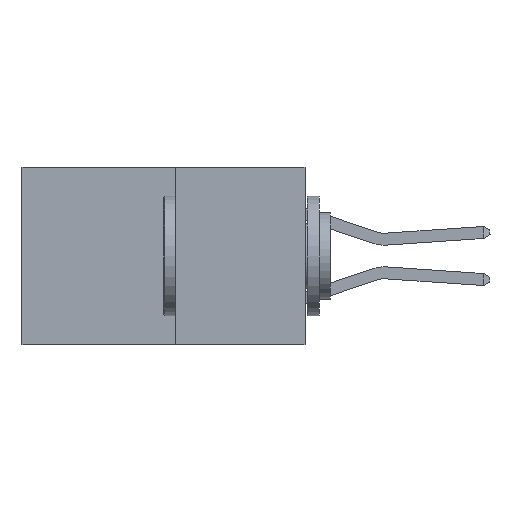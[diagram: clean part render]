
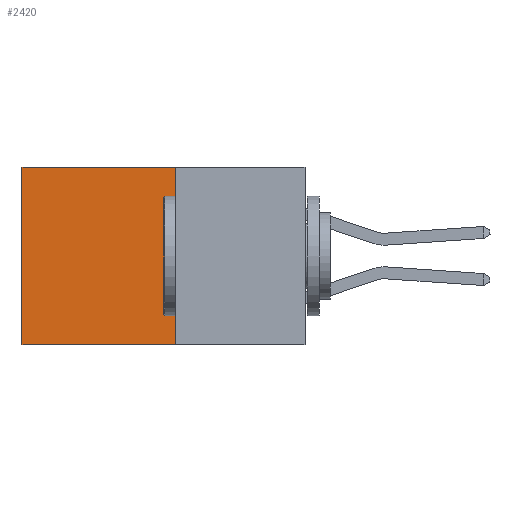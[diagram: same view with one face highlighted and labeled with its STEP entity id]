
A CAD part, left-side view. The second image highlights one B-rep face of the part: STEP entity #2420.
In plain terms, the highlighted planar face has unit normal (-1, 0, 0).
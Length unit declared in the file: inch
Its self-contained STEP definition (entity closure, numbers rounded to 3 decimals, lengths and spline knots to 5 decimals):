
#231 = CARTESIAN_POINT ( 'NONE',  ( 0.277, 0.27, 0. ) ) ;
#305 = LINE ( 'NONE', #4932, #8476 ) ;
#580 = DIRECTION ( 'NONE',  ( 0., 1., 0. ) ) ;
#593 = ORIENTED_EDGE ( 'NONE', *, *, #9528, .F. ) ;
#755 = DIRECTION ( 'NONE',  ( 0., 1., 0. ) ) ;
#769 = CARTESIAN_POINT ( 'NONE',  ( 0.277, 0.27, -0.37 ) ) ;
#1310 = CARTESIAN_POINT ( 'NONE',  ( 0.277, 0.27, -0.37 ) ) ;
#2315 = FACE_OUTER_BOUND ( 'NONE', #2800, .T. ) ;
#2420 = ADVANCED_FACE ( 'NONE', ( #2315 ), #5963, .F. ) ;
#2690 = LINE ( 'NONE', #1310, #4550 ) ;
#2800 = EDGE_LOOP ( 'NONE', ( #2806, #593, #2823, #6889 ) ) ;
#2801 = EDGE_CURVE ( 'NONE', #5486, #8533, #305, .T. ) ;
#2806 = ORIENTED_EDGE ( 'NONE', *, *, #2801, .T. ) ;
#2823 = ORIENTED_EDGE ( 'NONE', *, *, #6991, .F. ) ;
#3002 = VECTOR ( 'NONE', #580, 39.37008 ) ;
#3126 = DIRECTION ( 'NONE',  ( 0., 0., -1. ) ) ;
#3363 = DIRECTION ( 'NONE',  ( 0., 0., -1. ) ) ;
#3521 = CARTESIAN_POINT ( 'NONE',  ( 0.277, 0.59, 0. ) ) ;
#3761 = CARTESIAN_POINT ( 'NONE',  ( 0.277, 0.59, -0.37 ) ) ;
#3811 = EDGE_CURVE ( 'NONE', #9253, #5486, #9293, .T. ) ;
#4550 = VECTOR ( 'NONE', #3126, 39.37008 ) ;
#4932 = CARTESIAN_POINT ( 'NONE',  ( 0.277, 0.59, -0.37 ) ) ;
#5310 = DIRECTION ( 'NONE',  ( 0., 0., -1. ) ) ;
#5486 = VERTEX_POINT ( 'NONE', #3521 ) ;
#5963 = PLANE ( 'NONE',  #9778 ) ;
#6267 = VERTEX_POINT ( 'NONE', #8669 ) ;
#6889 = ORIENTED_EDGE ( 'NONE', *, *, #3811, .T. ) ;
#6991 = EDGE_CURVE ( 'NONE', #9253, #6267, #2690, .T. ) ;
#7345 = VECTOR ( 'NONE', #755, 39.37008 ) ;
#7564 = CARTESIAN_POINT ( 'NONE',  ( 0.277, 0.27, 0. ) ) ;
#7847 = LINE ( 'NONE', #769, #7345 ) ;
#8476 = VECTOR ( 'NONE', #5310, 39.37008 ) ;
#8533 = VERTEX_POINT ( 'NONE', #3761 ) ;
#8669 = CARTESIAN_POINT ( 'NONE',  ( 0.277, 0.27, -0.37 ) ) ;
#9253 = VERTEX_POINT ( 'NONE', #7564 ) ;
#9293 = LINE ( 'NONE', #231, #3002 ) ;
#9470 = DIRECTION ( 'NONE',  ( 1., 0., 0. ) ) ;
#9528 = EDGE_CURVE ( 'NONE', #6267, #8533, #7847, .T. ) ;
#9614 = CARTESIAN_POINT ( 'NONE',  ( 0.277, 0.27, -0.37 ) ) ;
#9778 = AXIS2_PLACEMENT_3D ( 'NONE', #9614, #9470, #3363 ) ;
